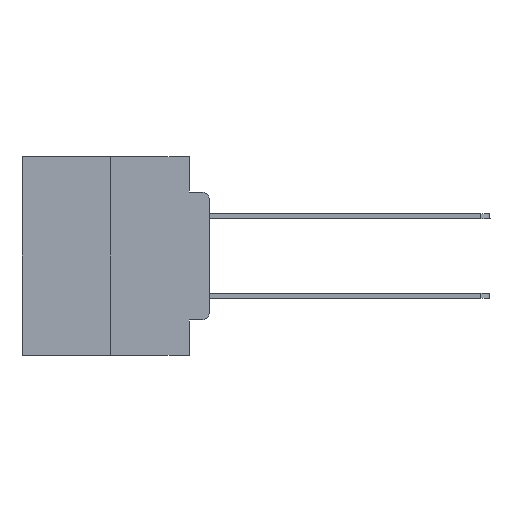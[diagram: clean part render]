
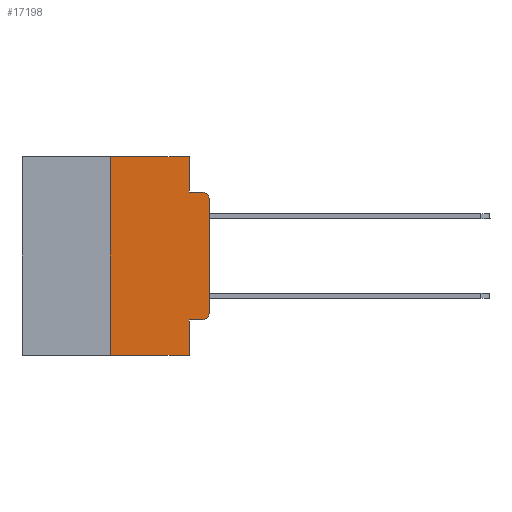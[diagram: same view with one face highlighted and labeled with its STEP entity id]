
A CAD part, left-side view. The second image highlights one B-rep face of the part: STEP entity #17198.
In plain terms, the highlighted planar face has unit normal (-1, 0, 0).
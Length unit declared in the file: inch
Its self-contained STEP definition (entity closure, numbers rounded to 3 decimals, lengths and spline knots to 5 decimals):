
#224 = VERTEX_POINT ( 'NONE', #2800 ) ;
#423 = CARTESIAN_POINT ( 'NONE',  ( 0., 0., 0. ) ) ;
#974 = DIRECTION ( 'NONE',  ( -1., 0., 0. ) ) ;
#1146 = VECTOR ( 'NONE', #15557, 39.37008 ) ;
#1491 = AXIS2_PLACEMENT_3D ( 'NONE', #23120, #3576, #3748 ) ;
#1666 = ORIENTED_EDGE ( 'NONE', *, *, #21169, .T. ) ;
#1800 = EDGE_CURVE ( 'NONE', #20195, #22870, #21664, .T. ) ;
#2800 = CARTESIAN_POINT ( 'NONE',  ( 0., 0., -0.3915 ) ) ;
#3255 = DIRECTION ( 'NONE',  ( 0., 0., -1. ) ) ;
#3368 = VECTOR ( 'NONE', #15451, 39.37008 ) ;
#3576 = DIRECTION ( 'NONE',  ( 1., 0., 0. ) ) ;
#3748 = DIRECTION ( 'NONE',  ( 0., 0., -1. ) ) ;
#4190 = DIRECTION ( 'NONE',  ( 0., 0., -1. ) ) ;
#4257 = VECTOR ( 'NONE', #12532, 39.37008 ) ;
#4420 = CIRCLE ( 'NONE', #22751, 0.02 ) ;
#4975 = ORIENTED_EDGE ( 'NONE', *, *, #7251, .F. ) ;
#5164 = CARTESIAN_POINT ( 'NONE',  ( 0., 0.02, -0.4115 ) ) ;
#5385 = CARTESIAN_POINT ( 'NONE',  ( 0., 0.051, 0. ) ) ;
#5878 = VECTOR ( 'NONE', #22954, 39.37008 ) ;
#5980 = VECTOR ( 'NONE', #8915, 39.37008 ) ;
#6047 = DIRECTION ( 'NONE',  ( -1., 0., 0. ) ) ;
#6217 = LINE ( 'NONE', #9029, #21645 ) ;
#7077 = DIRECTION ( 'NONE',  ( 0., -1., 0. ) ) ;
#7083 = EDGE_CURVE ( 'NONE', #10203, #21299, #11607, .T. ) ;
#7116 = AXIS2_PLACEMENT_3D ( 'NONE', #20550, #974, #3255 ) ;
#7251 = EDGE_CURVE ( 'NONE', #9663, #24393, #15941, .T. ) ;
#8224 = ORIENTED_EDGE ( 'NONE', *, *, #1800, .F. ) ;
#8383 = LINE ( 'NONE', #423, #3368 ) ;
#8667 = DIRECTION ( 'NONE',  ( 0., -1., 0. ) ) ;
#8915 = DIRECTION ( 'NONE',  ( 0., -1., 0. ) ) ;
#9013 = VECTOR ( 'NONE', #7077, 39.37008 ) ;
#9029 = CARTESIAN_POINT ( 'NONE',  ( 0., 0.473, -0.5 ) ) ;
#9324 = CARTESIAN_POINT ( 'NONE',  ( 0., 0.25, -0.5 ) ) ;
#9422 = CARTESIAN_POINT ( 'NONE',  ( 0., 0.051, -0.4115 ) ) ;
#9655 = EDGE_CURVE ( 'NONE', #22154, #224, #23789, .T. ) ;
#9663 = VERTEX_POINT ( 'NONE', #5385 ) ;
#10203 = VERTEX_POINT ( 'NONE', #9324 ) ;
#10206 = VERTEX_POINT ( 'NONE', #20065 ) ;
#11405 = CARTESIAN_POINT ( 'NONE',  ( 0., 0.473, 0. ) ) ;
#11537 = ORIENTED_EDGE ( 'NONE', *, *, #14141, .F. ) ;
#11607 = LINE ( 'NONE', #22856, #5878 ) ;
#12035 = LINE ( 'NONE', #11405, #9013 ) ;
#12065 = CARTESIAN_POINT ( 'NONE',  ( 0., 0.051, -0.0885 ) ) ;
#12510 = VECTOR ( 'NONE', #18694, 39.37008 ) ;
#12532 = DIRECTION ( 'NONE',  ( 0., 0., -1. ) ) ;
#13012 = CARTESIAN_POINT ( 'NONE',  ( 0., 0.25, 0. ) ) ;
#13137 = CARTESIAN_POINT ( 'NONE',  ( 0., 0.051, 0. ) ) ;
#13144 = ORIENTED_EDGE ( 'NONE', *, *, #23187, .F. ) ;
#14083 = EDGE_LOOP ( 'NONE', ( #27704, #1666, #11537, #4975, #13144, #21119, #15120, #8224, #14166, #17581 ) ) ;
#14141 = EDGE_CURVE ( 'NONE', #24393, #19798, #20200, .T. ) ;
#14166 = ORIENTED_EDGE ( 'NONE', *, *, #24120, .T. ) ;
#14699 = CARTESIAN_POINT ( 'NONE',  ( 0., 0.02, -0.1085 ) ) ;
#15120 = ORIENTED_EDGE ( 'NONE', *, *, #25242, .T. ) ;
#15451 = DIRECTION ( 'NONE',  ( 0., 0., 1. ) ) ;
#15557 = DIRECTION ( 'NONE',  ( 0., 0., -1. ) ) ;
#15941 = LINE ( 'NONE', #13137, #1146 ) ;
#16293 = CARTESIAN_POINT ( 'NONE',  ( 0., 0.02, -0.0885 ) ) ;
#17198 = ADVANCED_FACE ( 'NONE', ( #18670 ), #18742, .F. ) ;
#17581 = ORIENTED_EDGE ( 'NONE', *, *, #9655, .T. ) ;
#18670 = FACE_OUTER_BOUND ( 'NONE', #14083, .T. ) ;
#18694 = DIRECTION ( 'NONE',  ( 0., -1., 0. ) ) ;
#18742 = PLANE ( 'NONE',  #1491 ) ;
#19071 = LINE ( 'NONE', #22704, #5980 ) ;
#19798 = VERTEX_POINT ( 'NONE', #16293 ) ;
#20065 = CARTESIAN_POINT ( 'NONE',  ( 0., 0., -0.1085 ) ) ;
#20195 = VERTEX_POINT ( 'NONE', #9422 ) ;
#20200 = LINE ( 'NONE', #12065, #12510 ) ;
#20550 = CARTESIAN_POINT ( 'NONE',  ( 0., 0.02, -0.3915 ) ) ;
#21034 = CARTESIAN_POINT ( 'NONE',  ( 0., 0.051, -0.0885 ) ) ;
#21119 = ORIENTED_EDGE ( 'NONE', *, *, #7083, .F. ) ;
#21169 = EDGE_CURVE ( 'NONE', #10206, #19798, #4420, .T. ) ;
#21299 = VERTEX_POINT ( 'NONE', #13012 ) ;
#21390 = CARTESIAN_POINT ( 'NONE',  ( 0., 0.051, 0. ) ) ;
#21645 = VECTOR ( 'NONE', #8667, 39.37008 ) ;
#21664 = LINE ( 'NONE', #21390, #4257 ) ;
#22154 = VERTEX_POINT ( 'NONE', #5164 ) ;
#22659 = EDGE_CURVE ( 'NONE', #224, #10206, #8383, .T. ) ;
#22704 = CARTESIAN_POINT ( 'NONE',  ( 0., 0.051, -0.4115 ) ) ;
#22751 = AXIS2_PLACEMENT_3D ( 'NONE', #14699, #6047, #4190 ) ;
#22856 = CARTESIAN_POINT ( 'NONE',  ( 0., 0.25, 0. ) ) ;
#22870 = VERTEX_POINT ( 'NONE', #27498 ) ;
#22954 = DIRECTION ( 'NONE',  ( 0., 0., 1. ) ) ;
#23120 = CARTESIAN_POINT ( 'NONE',  ( 0., 0.473, 0. ) ) ;
#23187 = EDGE_CURVE ( 'NONE', #21299, #9663, #12035, .T. ) ;
#23789 = CIRCLE ( 'NONE', #7116, 0.02 ) ;
#24120 = EDGE_CURVE ( 'NONE', #20195, #22154, #19071, .T. ) ;
#24393 = VERTEX_POINT ( 'NONE', #21034 ) ;
#25242 = EDGE_CURVE ( 'NONE', #10203, #22870, #6217, .T. ) ;
#27498 = CARTESIAN_POINT ( 'NONE',  ( 0., 0.051, -0.5 ) ) ;
#27704 = ORIENTED_EDGE ( 'NONE', *, *, #22659, .T. ) ;
